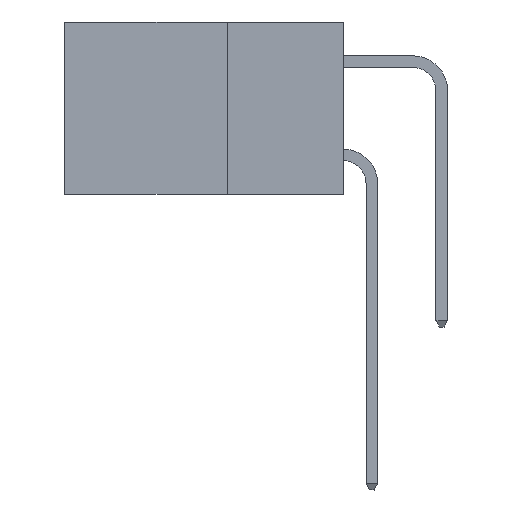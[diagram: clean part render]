
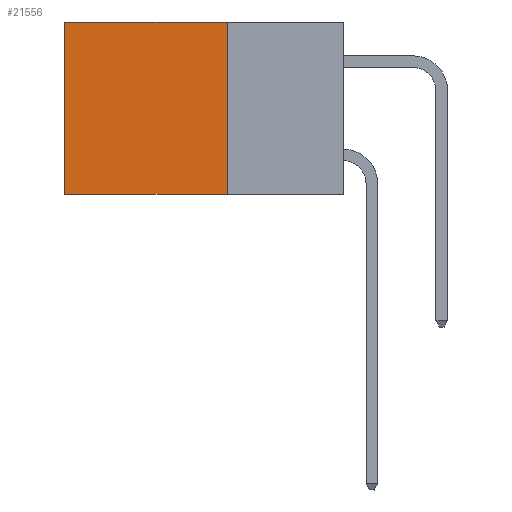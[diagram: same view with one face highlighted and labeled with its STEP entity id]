
A CAD part, left-side view. The second image highlights one B-rep face of the part: STEP entity #21556.
In plain terms, the highlighted planar face has unit normal (-1, 0, 0).
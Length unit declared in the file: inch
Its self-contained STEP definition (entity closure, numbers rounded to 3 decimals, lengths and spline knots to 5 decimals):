
#740 = LINE ( 'NONE', #23047, #1505 ) ;
#1459 = LINE ( 'NONE', #22456, #7917 ) ;
#1505 = VECTOR ( 'NONE', #25422, 39.37008 ) ;
#2395 = VERTEX_POINT ( 'NONE', #15259 ) ;
#3082 = DIRECTION ( 'NONE',  ( 0., 1., 0. ) ) ;
#5917 = ORIENTED_EDGE ( 'NONE', *, *, #15996, .F. ) ;
#6342 = VERTEX_POINT ( 'NONE', #27831 ) ;
#6386 = CARTESIAN_POINT ( 'NONE',  ( 0.298, 0.25, 0. ) ) ;
#7917 = VECTOR ( 'NONE', #3082, 39.37008 ) ;
#8821 = DIRECTION ( 'NONE',  ( 1., 0., 0. ) ) ;
#8947 = DIRECTION ( 'NONE',  ( 0., 1., 0. ) ) ;
#10256 = ORIENTED_EDGE ( 'NONE', *, *, #22174, .T. ) ;
#10431 = ORIENTED_EDGE ( 'NONE', *, *, #19728, .T. ) ;
#11345 = FACE_OUTER_BOUND ( 'NONE', #17726, .T. ) ;
#11347 = AXIS2_PLACEMENT_3D ( 'NONE', #6386, #8821, #25660 ) ;
#12247 = VECTOR ( 'NONE', #30333, 39.37008 ) ;
#14614 = VERTEX_POINT ( 'NONE', #25468 ) ;
#15259 = CARTESIAN_POINT ( 'NONE',  ( 0.298, 0.6, -0.37 ) ) ;
#15996 = EDGE_CURVE ( 'NONE', #14614, #6342, #25104, .T. ) ;
#16502 = ORIENTED_EDGE ( 'NONE', *, *, #19424, .F. ) ;
#17726 = EDGE_LOOP ( 'NONE', ( #10256, #16502, #5917, #10431 ) ) ;
#19424 = EDGE_CURVE ( 'NONE', #6342, #2395, #23436, .T. ) ;
#19728 = EDGE_CURVE ( 'NONE', #14614, #27066, #1459, .T. ) ;
#20885 = PLANE ( 'NONE',  #11347 ) ;
#21556 = ADVANCED_FACE ( 'NONE', ( #11345 ), #20885, .F. ) ;
#22144 = CARTESIAN_POINT ( 'NONE',  ( 0.298, 0.6, 0. ) ) ;
#22174 = EDGE_CURVE ( 'NONE', #27066, #2395, #740, .T. ) ;
#22456 = CARTESIAN_POINT ( 'NONE',  ( 0.298, 0.25, 0. ) ) ;
#22698 = VECTOR ( 'NONE', #8947, 39.37008 ) ;
#23047 = CARTESIAN_POINT ( 'NONE',  ( 0.298, 0.6, 0. ) ) ;
#23218 = CARTESIAN_POINT ( 'NONE',  ( 0.298, 0.25, 0. ) ) ;
#23436 = LINE ( 'NONE', #25779, #22698 ) ;
#25104 = LINE ( 'NONE', #23218, #12247 ) ;
#25422 = DIRECTION ( 'NONE',  ( 0., 0., -1. ) ) ;
#25468 = CARTESIAN_POINT ( 'NONE',  ( 0.298, 0.25, 0. ) ) ;
#25660 = DIRECTION ( 'NONE',  ( 0., 0., -1. ) ) ;
#25779 = CARTESIAN_POINT ( 'NONE',  ( 0.298, 0.25, -0.37 ) ) ;
#27066 = VERTEX_POINT ( 'NONE', #22144 ) ;
#27831 = CARTESIAN_POINT ( 'NONE',  ( 0.298, 0.25, -0.37 ) ) ;
#30333 = DIRECTION ( 'NONE',  ( 0., 0., -1. ) ) ;
